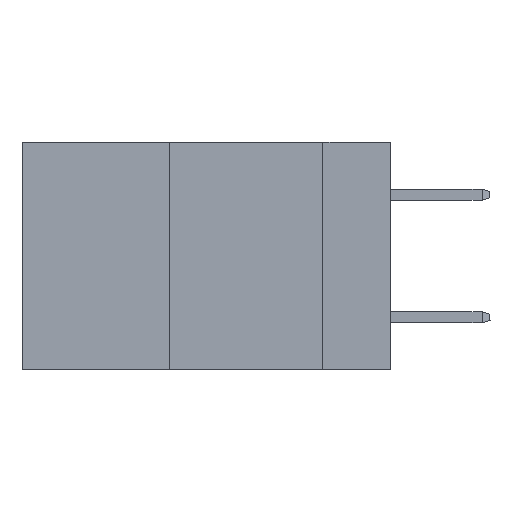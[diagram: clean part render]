
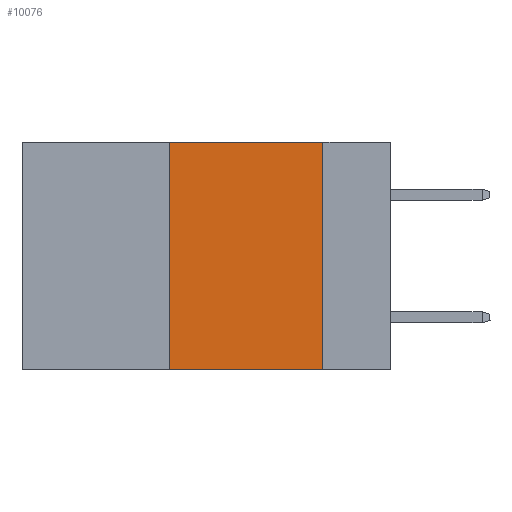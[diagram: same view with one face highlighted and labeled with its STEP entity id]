
A CAD part, left-side view. The second image highlights one B-rep face of the part: STEP entity #10076.
In plain terms, the highlighted planar face has unit normal (-1, 0, 0).
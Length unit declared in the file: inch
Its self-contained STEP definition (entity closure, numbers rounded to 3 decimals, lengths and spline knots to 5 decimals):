
#242 = DIRECTION ( 'NONE',  ( 1., 0., 0. ) ) ;
#1023 = EDGE_CURVE ( 'NONE', #2961, #7058, #12699, .T. ) ;
#2215 = CARTESIAN_POINT ( 'NONE',  ( 0., 0.6, 0. ) ) ;
#2961 = VERTEX_POINT ( 'NONE', #10550 ) ;
#2968 = CARTESIAN_POINT ( 'NONE',  ( 0., 0.11, 0. ) ) ;
#3645 = ORIENTED_EDGE ( 'NONE', *, *, #10202, .F. ) ;
#4835 = LINE ( 'NONE', #2215, #7599 ) ;
#5150 = ORIENTED_EDGE ( 'NONE', *, *, #8629, .T. ) ;
#6726 = VECTOR ( 'NONE', #13021, 39.37008 ) ;
#6764 = VERTEX_POINT ( 'NONE', #8723 ) ;
#6766 = VECTOR ( 'NONE', #8917, 39.37008 ) ;
#7058 = VERTEX_POINT ( 'NONE', #14056 ) ;
#7456 = LINE ( 'NONE', #8288, #6726 ) ;
#7484 = PLANE ( 'NONE',  #10123 ) ;
#7599 = VECTOR ( 'NONE', #8137, 39.37008 ) ;
#8137 = DIRECTION ( 'NONE',  ( 0., -1., 0. ) ) ;
#8153 = VERTEX_POINT ( 'NONE', #12189 ) ;
#8288 = CARTESIAN_POINT ( 'NONE',  ( 0., 0.6, -0.37 ) ) ;
#8629 = EDGE_CURVE ( 'NONE', #2961, #6764, #7456, .T. ) ;
#8641 = DIRECTION ( 'NONE',  ( 0., 0., -1. ) ) ;
#8723 = CARTESIAN_POINT ( 'NONE',  ( 0., 0.11, -0.37 ) ) ;
#8907 = CARTESIAN_POINT ( 'NONE',  ( 0., 0.36, 0. ) ) ;
#8917 = DIRECTION ( 'NONE',  ( 0., 0., 1. ) ) ;
#9701 = FACE_OUTER_BOUND ( 'NONE', #13259, .T. ) ;
#9905 = ORIENTED_EDGE ( 'NONE', *, *, #13876, .F. ) ;
#10027 = DIRECTION ( 'NONE',  ( 0., 0., -1. ) ) ;
#10076 = ADVANCED_FACE ( 'NONE', ( #9701 ), #7484, .F. ) ;
#10123 = AXIS2_PLACEMENT_3D ( 'NONE', #14581, #242, #8641 ) ;
#10202 = EDGE_CURVE ( 'NONE', #8153, #6764, #10976, .T. ) ;
#10275 = ORIENTED_EDGE ( 'NONE', *, *, #1023, .F. ) ;
#10550 = CARTESIAN_POINT ( 'NONE',  ( 0., 0.36, -0.37 ) ) ;
#10608 = VECTOR ( 'NONE', #10027, 39.37008 ) ;
#10976 = LINE ( 'NONE', #2968, #10608 ) ;
#12189 = CARTESIAN_POINT ( 'NONE',  ( 0., 0.11, 0. ) ) ;
#12699 = LINE ( 'NONE', #8907, #6766 ) ;
#13021 = DIRECTION ( 'NONE',  ( 0., -1., 0. ) ) ;
#13259 = EDGE_LOOP ( 'NONE', ( #3645, #9905, #10275, #5150 ) ) ;
#13876 = EDGE_CURVE ( 'NONE', #7058, #8153, #4835, .T. ) ;
#14056 = CARTESIAN_POINT ( 'NONE',  ( 0., 0.36, 0. ) ) ;
#14581 = CARTESIAN_POINT ( 'NONE',  ( 0., 0.6, 0. ) ) ;
